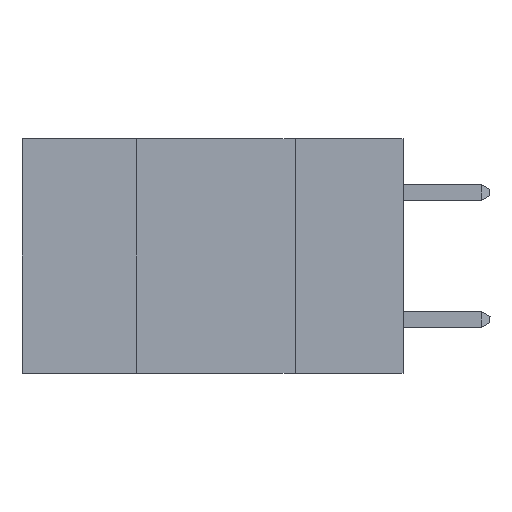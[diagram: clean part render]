
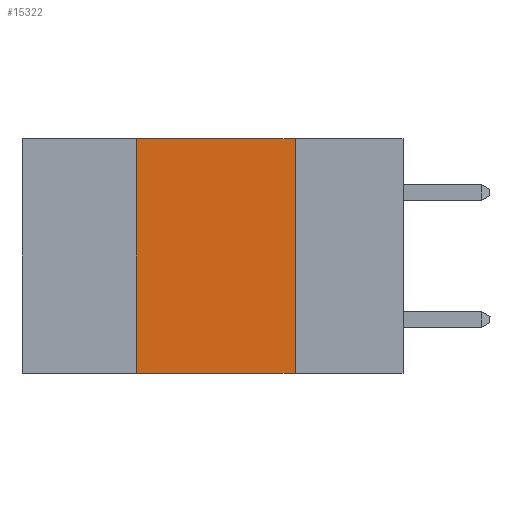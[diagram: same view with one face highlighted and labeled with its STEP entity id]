
A CAD part, left-side view. The second image highlights one B-rep face of the part: STEP entity #15322.
In plain terms, the highlighted planar face has unit normal (-1, 0, 0).
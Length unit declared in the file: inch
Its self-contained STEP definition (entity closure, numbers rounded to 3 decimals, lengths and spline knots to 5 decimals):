
#18 = EDGE_LOOP ( 'NONE', ( #35, #1823, #11460, #11111 ) ) ;
#35 = ORIENTED_EDGE ( 'NONE', *, *, #10789, .F. ) ;
#447 = LINE ( 'NONE', #7515, #14066 ) ;
#1070 = DIRECTION ( 'NONE',  ( 0., -1., 0. ) ) ;
#1240 = CARTESIAN_POINT ( 'NONE',  ( 0., 0.17, -0.37 ) ) ;
#1640 = VECTOR ( 'NONE', #13605, 39.37008 ) ;
#1823 = ORIENTED_EDGE ( 'NONE', *, *, #6214, .F. ) ;
#3142 = CARTESIAN_POINT ( 'NONE',  ( 0., 0.42, -0.37 ) ) ;
#4052 = CARTESIAN_POINT ( 'NONE',  ( 0., 0.6, -0.37 ) ) ;
#4296 = LINE ( 'NONE', #4052, #1640 ) ;
#5162 = VERTEX_POINT ( 'NONE', #10421 ) ;
#6214 = EDGE_CURVE ( 'NONE', #5162, #11788, #9078, .T. ) ;
#6764 = DIRECTION ( 'NONE',  ( 0., 0., -1. ) ) ;
#6990 = EDGE_CURVE ( 'NONE', #14783, #11871, #4296, .T. ) ;
#7344 = EDGE_CURVE ( 'NONE', #14783, #5162, #447, .T. ) ;
#7515 = CARTESIAN_POINT ( 'NONE',  ( 0., 0.42, 0. ) ) ;
#9032 = PLANE ( 'NONE',  #14171 ) ;
#9078 = LINE ( 'NONE', #11425, #12300 ) ;
#9265 = DIRECTION ( 'NONE',  ( 1., 0., 0. ) ) ;
#10381 = DIRECTION ( 'NONE',  ( 0., 0., -1. ) ) ;
#10421 = CARTESIAN_POINT ( 'NONE',  ( 0., 0.42, 0. ) ) ;
#10789 = EDGE_CURVE ( 'NONE', #11788, #11871, #12710, .T. ) ;
#10948 = CARTESIAN_POINT ( 'NONE',  ( 0., 0.17, 0. ) ) ;
#11111 = ORIENTED_EDGE ( 'NONE', *, *, #6990, .T. ) ;
#11411 = CARTESIAN_POINT ( 'NONE',  ( 0., 0.17, 0. ) ) ;
#11425 = CARTESIAN_POINT ( 'NONE',  ( 0., 0.6, 0. ) ) ;
#11458 = FACE_OUTER_BOUND ( 'NONE', #18, .T. ) ;
#11460 = ORIENTED_EDGE ( 'NONE', *, *, #7344, .F. ) ;
#11788 = VERTEX_POINT ( 'NONE', #10948 ) ;
#11871 = VERTEX_POINT ( 'NONE', #1240 ) ;
#12300 = VECTOR ( 'NONE', #1070, 39.37008 ) ;
#12366 = VECTOR ( 'NONE', #10381, 39.37008 ) ;
#12576 = DIRECTION ( 'NONE',  ( 0., 0., 1. ) ) ;
#12710 = LINE ( 'NONE', #11411, #12366 ) ;
#13605 = DIRECTION ( 'NONE',  ( 0., -1., 0. ) ) ;
#13759 = CARTESIAN_POINT ( 'NONE',  ( 0., 0.6, 0. ) ) ;
#14066 = VECTOR ( 'NONE', #12576, 39.37008 ) ;
#14171 = AXIS2_PLACEMENT_3D ( 'NONE', #13759, #9265, #6764 ) ;
#14783 = VERTEX_POINT ( 'NONE', #3142 ) ;
#15322 = ADVANCED_FACE ( 'NONE', ( #11458 ), #9032, .F. ) ;
